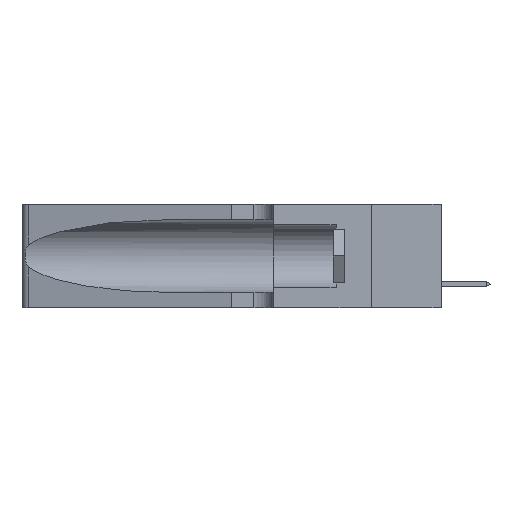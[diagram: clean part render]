
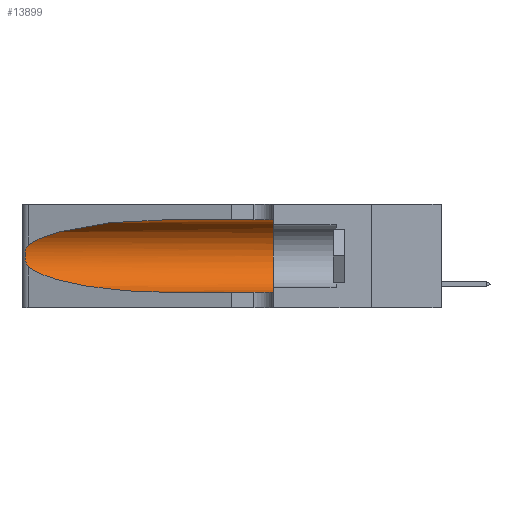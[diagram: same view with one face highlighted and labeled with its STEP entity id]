
A CAD part, left-side view. The second image highlights one B-rep face of the part: STEP entity #13899.
In plain terms, the highlighted cylindrical face has radius 3.308 mm (diameter 6.617 mm), a partial arc.
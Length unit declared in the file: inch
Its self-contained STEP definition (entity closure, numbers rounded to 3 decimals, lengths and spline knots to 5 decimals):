
#489 = DIRECTION ( 'NONE',  ( 0., -1., 0. ) ) ;
#1365 = EDGE_CURVE ( 'NONE', #13900, #47310, #2922, .T. ) ;
#1837 = LINE ( 'NONE', #10901, #26818 ) ;
#1946 = EDGE_CURVE ( 'NONE', #47737, #36632, #1837, .T. ) ;
#2922 = LINE ( 'NONE', #34107, #16896 ) ;
#2998 =( BOUNDED_CURVE ( )  B_SPLINE_CURVE ( 3, ( #21162, #20812, #24576, #47115 ),
 .UNSPECIFIED., .F., .F. ) 
 B_SPLINE_CURVE_WITH_KNOTS ( ( 4, 4 ),
 ( 1.5708, 2.84003 ),
 .UNSPECIFIED. ) 
 CURVE ( )  GEOMETRIC_REPRESENTATION_ITEM ( )  RATIONAL_B_SPLINE_CURVE ( ( 1., 0.87, 0.87, 1. ) ) 
 REPRESENTATION_ITEM ( '' )  );
#3824 = EDGE_CURVE ( 'NONE', #38336, #29096, #45812, .T. ) ;
#3998 = CARTESIAN_POINT ( 'NONE',  ( 0.25487, 1.22718, 0.22369 ) ) ;
#4748 = DIRECTION ( 'NONE',  ( 0., 1., 0. ) ) ;
#6063 = CARTESIAN_POINT ( 'NONE',  ( 0.25487, 1.22718, 0.14631 ) ) ;
#6661 = AXIS2_PLACEMENT_3D ( 'NONE', #30114, #489, #26188 ) ;
#7124 = CARTESIAN_POINT ( 'NONE',  ( 0.2373, 1.15595, 0.08982 ) ) ;
#10901 = CARTESIAN_POINT ( 'NONE',  ( 0.1305, 1.61858, 0.05475 ) ) ;
#11143 = FACE_OUTER_BOUND ( 'NONE', #26780, .T. ) ;
#11542 = DIRECTION ( 'NONE',  ( 0., -1., 0. ) ) ;
#11748 = CARTESIAN_POINT ( 'NONE',  ( 0.1305, 0.35, 0.185 ) ) ;
#13899 = ADVANCED_FACE ( 'NONE', ( #11143 ), #14058, .F. ) ;
#13900 = VERTEX_POINT ( 'NONE', #26035 ) ;
#14058 = CYLINDRICAL_SURFACE ( 'NONE', #6661, 0.13025 ) ;
#14079 = CIRCLE ( 'NONE', #39308, 0.13025 ) ;
#16896 = VECTOR ( 'NONE', #35557, 39.37008 ) ;
#18245 = CARTESIAN_POINT ( 'NONE',  ( 0.25789, 1.23486, 0.15765 ) ) ;
#18321 = CARTESIAN_POINT ( 'NONE',  ( 0.18966, 0.96281, 0.05475 ) ) ;
#18549 = CARTESIAN_POINT ( 'NONE',  ( 0.25555, 1.22994, 0.2215 ) ) ;
#18885 = CARTESIAN_POINT ( 'NONE',  ( 0.25487, 1.22718, 0.22369 ) ) ;
#20812 = CARTESIAN_POINT ( 'NONE',  ( 0.18966, 0.96281, 0.31525 ) ) ;
#21162 = CARTESIAN_POINT ( 'NONE',  ( 0.1305, 0.72297, 0.31525 ) ) ;
#22055 = CARTESIAN_POINT ( 'NONE',  ( 0.1305, 0.72297, 0.05475 ) ) ;
#22148 = CARTESIAN_POINT ( 'NONE',  ( 0.26075, 1.23896, 0.19203 ) ) ;
#24576 = CARTESIAN_POINT ( 'NONE',  ( 0.2373, 1.15595, 0.28018 ) ) ;
#24865 = EDGE_CURVE ( 'NONE', #47310, #36632, #14079, .T. ) ;
#25557 = CARTESIAN_POINT ( 'NONE',  ( 0.25639, 1.23184, 0.21858 ) ) ;
#25906 = CARTESIAN_POINT ( 'NONE',  ( 0.25856, 1.23593, 0.16098 ) ) ;
#26035 = CARTESIAN_POINT ( 'NONE',  ( 0.1305, 0.72297, 0.31525 ) ) ;
#26049 = CARTESIAN_POINT ( 'NONE',  ( 0.25787, 1.23484, 0.2124 ) ) ;
#26188 = DIRECTION ( 'NONE',  ( 0., 0., -1. ) ) ;
#26780 = EDGE_LOOP ( 'NONE', ( #42402, #26835, #46448, #27670, #38497, #33900 ) ) ;
#26818 = VECTOR ( 'NONE', #11542, 39.37008 ) ;
#26835 = ORIENTED_EDGE ( 'NONE', *, *, #3824, .T. ) ;
#27670 = ORIENTED_EDGE ( 'NONE', *, *, #1946, .T. ) ;
#29096 = VERTEX_POINT ( 'NONE', #6063 ) ;
#29822 = CARTESIAN_POINT ( 'NONE',  ( 0.25555, 1.22993, 0.14849 ) ) ;
#30114 = CARTESIAN_POINT ( 'NONE',  ( 0.1305, 1.61858, 0.185 ) ) ;
#30748 = DIRECTION ( 'NONE',  ( 0., 0., 1. ) ) ;
#32494 =( BOUNDED_CURVE ( )  B_SPLINE_CURVE ( 3, ( #47523, #7124, #18321, #22055 ),
 .UNSPECIFIED., .F., .F. ) 
 B_SPLINE_CURVE_WITH_KNOTS ( ( 4, 4 ),
 ( 3.44316, 4.71239 ),
 .UNSPECIFIED. ) 
 CURVE ( )  GEOMETRIC_REPRESENTATION_ITEM ( )  RATIONAL_B_SPLINE_CURVE ( ( 1., 0.87, 0.87, 1. ) ) 
 REPRESENTATION_ITEM ( '' )  );
#33046 = CARTESIAN_POINT ( 'NONE',  ( 0.25854, 1.2359, 0.20912 ) ) ;
#33774 = EDGE_CURVE ( 'NONE', #29096, #47737, #32494, .T. ) ;
#33900 = ORIENTED_EDGE ( 'NONE', *, *, #1365, .F. ) ;
#33971 = CARTESIAN_POINT ( 'NONE',  ( 0.1305, 0.35, 0.05475 ) ) ;
#34107 = CARTESIAN_POINT ( 'NONE',  ( 0.1305, 1.61858, 0.31525 ) ) ;
#34894 = EDGE_CURVE ( 'NONE', #13900, #38336, #2998, .T. ) ;
#35557 = DIRECTION ( 'NONE',  ( 0., -1., 0. ) ) ;
#36632 = VERTEX_POINT ( 'NONE', #33971 ) ;
#36779 = CARTESIAN_POINT ( 'NONE',  ( 0.26018, 1.23835, 0.19895 ) ) ;
#38336 = VERTEX_POINT ( 'NONE', #3998 ) ;
#38497 = ORIENTED_EDGE ( 'NONE', *, *, #24865, .F. ) ;
#39308 = AXIS2_PLACEMENT_3D ( 'NONE', #11748, #4748, #30748 ) ;
#39518 = CARTESIAN_POINT ( 'NONE',  ( 0.1305, 0.72297, 0.05475 ) ) ;
#40497 = CARTESIAN_POINT ( 'NONE',  ( 0.26075, 1.23896, 0.178 ) ) ;
#40964 = CARTESIAN_POINT ( 'NONE',  ( 0.25487, 1.22718, 0.14631 ) ) ;
#42402 = ORIENTED_EDGE ( 'NONE', *, *, #34894, .T. ) ;
#44226 = CARTESIAN_POINT ( 'NONE',  ( 0.25639, 1.23186, 0.15144 ) ) ;
#44377 = CARTESIAN_POINT ( 'NONE',  ( 0.26017, 1.23833, 0.17102 ) ) ;
#45812 = B_SPLINE_CURVE_WITH_KNOTS ( 'NONE', 3,
 ( #18885, #18549, #25557, #26049, #33046, #36779, #22148, #40497, #44377, #25906, #18245, #44226, #29822, #40964 ),
 .UNSPECIFIED., .F., .F.,
 ( 4, 2, 2, 2, 2, 2, 4 ),
 ( 0., 0.00027, 0.00053, 0.00107, 0.0016, 0.00187, 0.00214 ),
 .UNSPECIFIED. ) ;
#46448 = ORIENTED_EDGE ( 'NONE', *, *, #33774, .T. ) ;
#47115 = CARTESIAN_POINT ( 'NONE',  ( 0.25487, 1.22718, 0.22369 ) ) ;
#47310 = VERTEX_POINT ( 'NONE', #47800 ) ;
#47523 = CARTESIAN_POINT ( 'NONE',  ( 0.25487, 1.22718, 0.14631 ) ) ;
#47737 = VERTEX_POINT ( 'NONE', #39518 ) ;
#47800 = CARTESIAN_POINT ( 'NONE',  ( 0.1305, 0.35, 0.31525 ) ) ;
